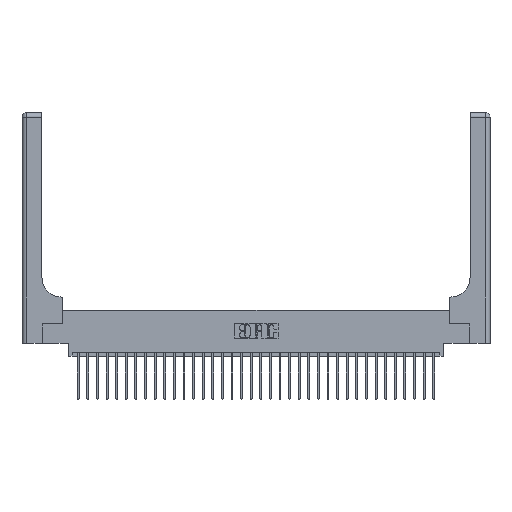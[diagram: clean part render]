
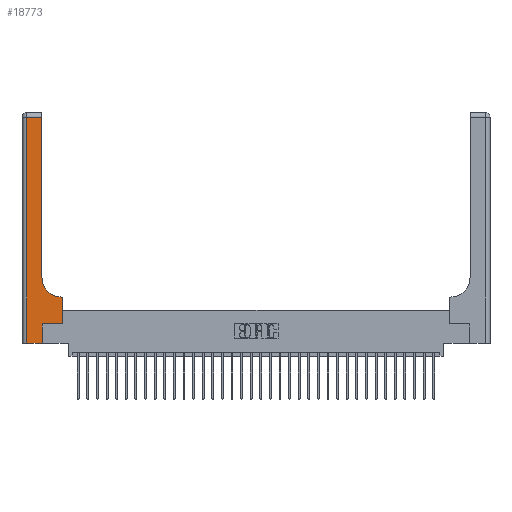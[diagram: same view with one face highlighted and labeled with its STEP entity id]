
A CAD part, top view. The second image highlights one B-rep face of the part: STEP entity #18773.
In plain terms, the highlighted planar face has unit normal (0, 0, 1).
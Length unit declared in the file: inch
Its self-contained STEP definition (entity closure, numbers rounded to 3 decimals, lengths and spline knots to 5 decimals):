
#616 = ORIENTED_EDGE ( 'NONE', *, *, #6634, .T. ) ;
#635 = LINE ( 'NONE', #8062, #4535 ) ;
#682 = CARTESIAN_POINT ( 'NONE',  ( 0.06, 2.94, 0.37 ) ) ;
#1191 = VERTEX_POINT ( 'NONE', #27015 ) ;
#1730 = CARTESIAN_POINT ( 'NONE',  ( 0.528, 0.25, 0.37 ) ) ;
#1879 = ORIENTED_EDGE ( 'NONE', *, *, #12343, .T. ) ;
#2554 = LINE ( 'NONE', #12184, #20234 ) ;
#3441 = ORIENTED_EDGE ( 'NONE', *, *, #6942, .T. ) ;
#4535 = VECTOR ( 'NONE', #12646, 39.37008 ) ;
#6634 = EDGE_CURVE ( 'NONE', #21443, #7899, #9476, .T. ) ;
#6942 = EDGE_CURVE ( 'NONE', #11795, #8511, #14392, .T. ) ;
#7246 = ORIENTED_EDGE ( 'NONE', *, *, #28160, .T. ) ;
#7291 = DIRECTION ( 'NONE',  ( -1., 0., 0. ) ) ;
#7603 = DIRECTION ( 'NONE',  ( 0., -1., 0. ) ) ;
#7760 = PLANE ( 'NONE',  #27463 ) ;
#7899 = VERTEX_POINT ( 'NONE', #11570 ) ;
#8006 = CARTESIAN_POINT ( 'NONE',  ( 0.51, 0.85, 0.37 ) ) ;
#8062 = CARTESIAN_POINT ( 'NONE',  ( 0.265, 0.25, 0.37 ) ) ;
#8511 = VERTEX_POINT ( 'NONE', #9729 ) ;
#8603 = DIRECTION ( 'NONE',  ( -1., 0., 0. ) ) ;
#9088 = LINE ( 'NONE', #16308, #18438 ) ;
#9417 = CARTESIAN_POINT ( 'NONE',  ( 0.51, 0.6, 0.37 ) ) ;
#9476 = LINE ( 'NONE', #1730, #17234 ) ;
#9529 = EDGE_CURVE ( 'NONE', #20204, #21443, #635, .T. ) ;
#9729 = CARTESIAN_POINT ( 'NONE',  ( 0.26, 0.85, 0.37 ) ) ;
#9742 = CARTESIAN_POINT ( 'NONE',  ( 0.265, 0., 0.37 ) ) ;
#10302 = FACE_OUTER_BOUND ( 'NONE', #12241, .T. ) ;
#11296 = EDGE_CURVE ( 'NONE', #8511, #1191, #21097, .T. ) ;
#11570 = CARTESIAN_POINT ( 'NONE',  ( 0.528, 0.6, 0.37 ) ) ;
#11687 = VECTOR ( 'NONE', #18744, 39.37008 ) ;
#11795 = VERTEX_POINT ( 'NONE', #9417 ) ;
#11926 = VERTEX_POINT ( 'NONE', #682 ) ;
#12157 = CARTESIAN_POINT ( 'NONE',  ( 0.26, 0.6, 0.37 ) ) ;
#12184 = CARTESIAN_POINT ( 'NONE',  ( 0.06, 3., 0.37 ) ) ;
#12241 = EDGE_LOOP ( 'NONE', ( #14763, #17920, #1879, #7246, #25456, #28232, #616, #30010, #3441 ) ) ;
#12343 = EDGE_CURVE ( 'NONE', #11926, #23586, #2554, .T. ) ;
#12646 = DIRECTION ( 'NONE',  ( 1., 0., 0. ) ) ;
#13867 = LINE ( 'NONE', #9742, #27383 ) ;
#13914 = CARTESIAN_POINT ( 'NONE',  ( 0.265, 0.25, 0.37 ) ) ;
#14296 = CARTESIAN_POINT ( 'NONE',  ( 0., 0., 0.37 ) ) ;
#14392 = CIRCLE ( 'NONE', #14408, 0.25 ) ;
#14408 = AXIS2_PLACEMENT_3D ( 'NONE', #8006, #17610, #29726 ) ;
#14537 = DIRECTION ( 'NONE',  ( -1., 0., 0. ) ) ;
#14763 = ORIENTED_EDGE ( 'NONE', *, *, #11296, .T. ) ;
#16308 = CARTESIAN_POINT ( 'NONE',  ( 0., 2.94, 0.37 ) ) ;
#16686 = EDGE_CURVE ( 'NONE', #30422, #20204, #13867, .T. ) ;
#17005 = VECTOR ( 'NONE', #14537, 39.37008 ) ;
#17234 = VECTOR ( 'NONE', #23475, 39.37008 ) ;
#17367 = CARTESIAN_POINT ( 'NONE',  ( 0., 3., 0.37 ) ) ;
#17610 = DIRECTION ( 'NONE',  ( 0., 0., -1. ) ) ;
#17920 = ORIENTED_EDGE ( 'NONE', *, *, #26738, .T. ) ;
#18438 = VECTOR ( 'NONE', #8603, 39.37008 ) ;
#18744 = DIRECTION ( 'NONE',  ( 0., 1., 0. ) ) ;
#18773 = ADVANCED_FACE ( 'NONE', ( #10302 ), #7760, .F. ) ;
#19879 = DIRECTION ( 'NONE',  ( 0., 0., -1. ) ) ;
#20204 = VERTEX_POINT ( 'NONE', #13914 ) ;
#20234 = VECTOR ( 'NONE', #7603, 39.37008 ) ;
#21092 = DIRECTION ( 'NONE',  ( 0., 1., 0. ) ) ;
#21097 = LINE ( 'NONE', #25511, #11687 ) ;
#21443 = VERTEX_POINT ( 'NONE', #30801 ) ;
#23475 = DIRECTION ( 'NONE',  ( 0., 1., 0. ) ) ;
#23586 = VERTEX_POINT ( 'NONE', #27934 ) ;
#23884 = DIRECTION ( 'NONE',  ( 1., 0., 0. ) ) ;
#25456 = ORIENTED_EDGE ( 'NONE', *, *, #16686, .T. ) ;
#25511 = CARTESIAN_POINT ( 'NONE',  ( 0.26, 3., 0.37 ) ) ;
#25546 = VECTOR ( 'NONE', #23884, 39.37008 ) ;
#26188 = LINE ( 'NONE', #12157, #17005 ) ;
#26251 = LINE ( 'NONE', #14296, #25546 ) ;
#26738 = EDGE_CURVE ( 'NONE', #1191, #11926, #9088, .T. ) ;
#27015 = CARTESIAN_POINT ( 'NONE',  ( 0.26, 2.94, 0.37 ) ) ;
#27383 = VECTOR ( 'NONE', #21092, 39.37008 ) ;
#27463 = AXIS2_PLACEMENT_3D ( 'NONE', #17367, #19879, #7291 ) ;
#27520 = CARTESIAN_POINT ( 'NONE',  ( 0.265, 0., 0.37 ) ) ;
#27934 = CARTESIAN_POINT ( 'NONE',  ( 0.06, 0., 0.37 ) ) ;
#28160 = EDGE_CURVE ( 'NONE', #23586, #30422, #26251, .T. ) ;
#28232 = ORIENTED_EDGE ( 'NONE', *, *, #9529, .T. ) ;
#28548 = EDGE_CURVE ( 'NONE', #7899, #11795, #26188, .T. ) ;
#29726 = DIRECTION ( 'NONE',  ( 1., 0., 0. ) ) ;
#30010 = ORIENTED_EDGE ( 'NONE', *, *, #28548, .T. ) ;
#30422 = VERTEX_POINT ( 'NONE', #27520 ) ;
#30801 = CARTESIAN_POINT ( 'NONE',  ( 0.528, 0.25, 0.37 ) ) ;
